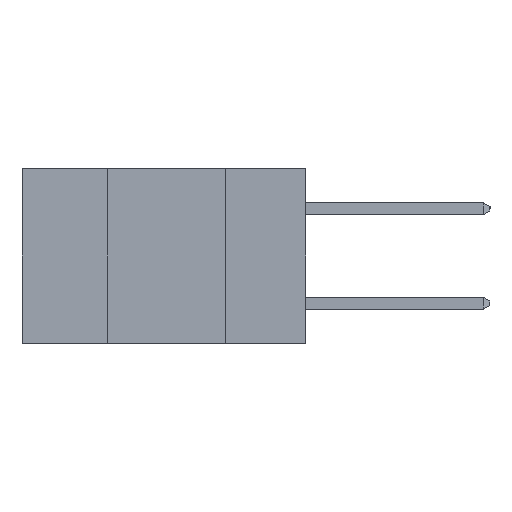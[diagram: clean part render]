
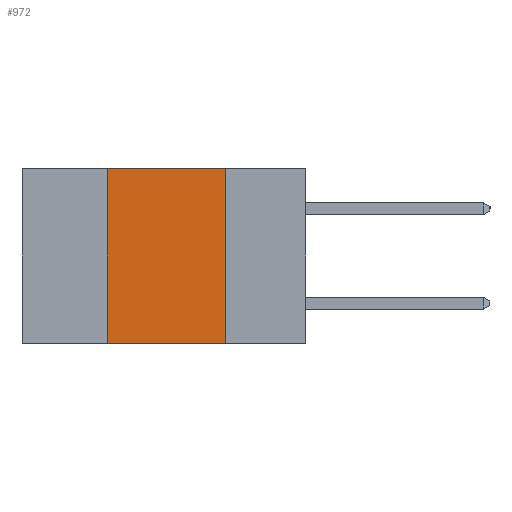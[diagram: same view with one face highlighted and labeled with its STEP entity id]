
A CAD part, left-side view. The second image highlights one B-rep face of the part: STEP entity #972.
In plain terms, the highlighted planar face has unit normal (-1, 0, 0).
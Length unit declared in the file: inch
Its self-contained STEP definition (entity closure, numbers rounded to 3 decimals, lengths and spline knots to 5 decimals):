
#178 = CARTESIAN_POINT ( 'NONE',  ( 0., 0.6, 0. ) ) ;
#383 = AXIS2_PLACEMENT_3D ( 'NONE', #7809, #1147, #4857 ) ;
#954 = EDGE_CURVE ( 'NONE', #2395, #3519, #7164, .T. ) ;
#972 = ADVANCED_FACE ( 'NONE', ( #7214 ), #5593, .F. ) ;
#1147 = DIRECTION ( 'NONE',  ( 1., 0., 0. ) ) ;
#1221 = DIRECTION ( 'NONE',  ( 0., 0., 1. ) ) ;
#1662 = EDGE_LOOP ( 'NONE', ( #5913, #7921, #3214, #2181 ) ) ;
#2181 = ORIENTED_EDGE ( 'NONE', *, *, #9302, .T. ) ;
#2395 = VERTEX_POINT ( 'NONE', #3723 ) ;
#2543 = CARTESIAN_POINT ( 'NONE',  ( 0., 0.17, -0.37 ) ) ;
#2916 = VERTEX_POINT ( 'NONE', #7398 ) ;
#3102 = LINE ( 'NONE', #3284, #7427 ) ;
#3155 = VECTOR ( 'NONE', #1221, 39.37008 ) ;
#3214 = ORIENTED_EDGE ( 'NONE', *, *, #5931, .F. ) ;
#3284 = CARTESIAN_POINT ( 'NONE',  ( 0., 0.6, -0.37 ) ) ;
#3519 = VERTEX_POINT ( 'NONE', #2543 ) ;
#3620 = EDGE_CURVE ( 'NONE', #2916, #2395, #7616, .T. ) ;
#3723 = CARTESIAN_POINT ( 'NONE',  ( 0., 0.17, 0. ) ) ;
#4381 = CARTESIAN_POINT ( 'NONE',  ( 0., 0.42, -0.37 ) ) ;
#4598 = VERTEX_POINT ( 'NONE', #8875 ) ;
#4857 = DIRECTION ( 'NONE',  ( 0., 0., -1. ) ) ;
#5452 = DIRECTION ( 'NONE',  ( 0., -1., 0. ) ) ;
#5593 = PLANE ( 'NONE',  #383 ) ;
#5913 = ORIENTED_EDGE ( 'NONE', *, *, #954, .F. ) ;
#5931 = EDGE_CURVE ( 'NONE', #4598, #2916, #8883, .T. ) ;
#6244 = DIRECTION ( 'NONE',  ( 0., -1., 0. ) ) ;
#6850 = VECTOR ( 'NONE', #7867, 39.37008 ) ;
#7164 = LINE ( 'NONE', #8707, #6850 ) ;
#7214 = FACE_OUTER_BOUND ( 'NONE', #1662, .T. ) ;
#7398 = CARTESIAN_POINT ( 'NONE',  ( 0., 0.42, 0. ) ) ;
#7427 = VECTOR ( 'NONE', #6244, 39.37008 ) ;
#7616 = LINE ( 'NONE', #178, #9689 ) ;
#7809 = CARTESIAN_POINT ( 'NONE',  ( 0., 0.6, 0. ) ) ;
#7867 = DIRECTION ( 'NONE',  ( 0., 0., -1. ) ) ;
#7921 = ORIENTED_EDGE ( 'NONE', *, *, #3620, .F. ) ;
#8707 = CARTESIAN_POINT ( 'NONE',  ( 0., 0.17, -0.37 ) ) ;
#8875 = CARTESIAN_POINT ( 'NONE',  ( 0., 0.42, -0.37 ) ) ;
#8883 = LINE ( 'NONE', #4381, #3155 ) ;
#9302 = EDGE_CURVE ( 'NONE', #4598, #3519, #3102, .T. ) ;
#9689 = VECTOR ( 'NONE', #5452, 39.37008 ) ;
